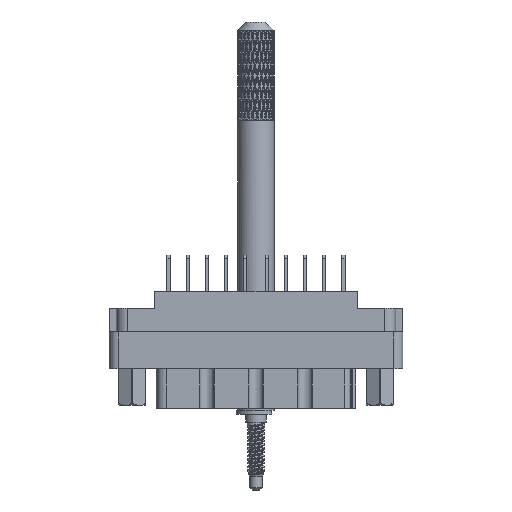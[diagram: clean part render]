
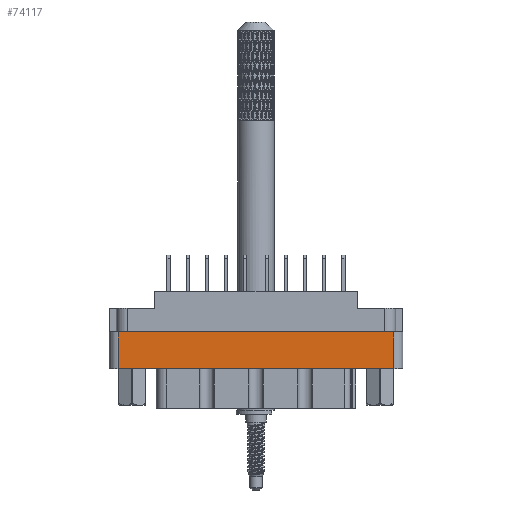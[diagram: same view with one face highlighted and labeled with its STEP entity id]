
A CAD part, front view. The second image highlights one B-rep face of the part: STEP entity #74117.
In plain terms, the highlighted planar face has unit normal (0, -1, 0).
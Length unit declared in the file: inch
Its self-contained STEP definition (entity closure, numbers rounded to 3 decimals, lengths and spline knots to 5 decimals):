
#2895 = VECTOR ( 'NONE', #45526, 39.37008 ) ;
#4321 = DIRECTION ( 'NONE',  ( 0., 0., -1. ) ) ;
#4507 = VERTEX_POINT ( 'NONE', #77688 ) ;
#5155 = CARTESIAN_POINT ( 'NONE',  ( 0.938, -0.438, -0.529 ) ) ;
#8470 = AXIS2_PLACEMENT_3D ( 'NONE', #83076, #100688, #4321 ) ;
#8472 = LINE ( 'NONE', #11501, #2895 ) ;
#9503 = VERTEX_POINT ( 'NONE', #14021 ) ;
#9946 = VERTEX_POINT ( 'NONE', #67772 ) ;
#11501 = CARTESIAN_POINT ( 'NONE',  ( 0., -0.438, -0.529 ) ) ;
#11908 = ORIENTED_EDGE ( 'NONE', *, *, #100642, .F. ) ;
#13003 = DIRECTION ( 'NONE',  ( 1., 0., 0. ) ) ;
#13657 = CARTESIAN_POINT ( 'NONE',  ( 0.938, -0.438, -0.798 ) ) ;
#13785 = CARTESIAN_POINT ( 'NONE',  ( 0., -0.438, -0.277 ) ) ;
#14021 = CARTESIAN_POINT ( 'NONE',  ( 0.938, -0.438, -0.277 ) ) ;
#21577 = PLANE ( 'NONE',  #8470 ) ;
#41378 = FACE_OUTER_BOUND ( 'NONE', #76787, .T. ) ;
#44194 = VECTOR ( 'NONE', #52657, 39.37008 ) ;
#45526 = DIRECTION ( 'NONE',  ( -1., 0., 0. ) ) ;
#49518 = CARTESIAN_POINT ( 'NONE',  ( -0.938, -0.438, -0.798 ) ) ;
#52657 = DIRECTION ( 'NONE',  ( 0., 0., -1. ) ) ;
#55251 = ORIENTED_EDGE ( 'NONE', *, *, #63183, .T. ) ;
#59979 = VECTOR ( 'NONE', #67132, 39.37008 ) ;
#63183 = EDGE_CURVE ( 'NONE', #88322, #9503, #99477, .T. ) ;
#67132 = DIRECTION ( 'NONE',  ( 0., 0., 1. ) ) ;
#67772 = CARTESIAN_POINT ( 'NONE',  ( -0.938, -0.438, -0.277 ) ) ;
#74117 = ADVANCED_FACE ( 'NONE', ( #41378 ), #21577, .T. ) ;
#76787 = EDGE_LOOP ( 'NONE', ( #11908, #105255, #108113, #55251 ) ) ;
#77688 = CARTESIAN_POINT ( 'NONE',  ( -0.938, -0.438, -0.529 ) ) ;
#82447 = LINE ( 'NONE', #49518, #44194 ) ;
#83076 = CARTESIAN_POINT ( 'NONE',  ( -1., -0.438, -0.798 ) ) ;
#83895 = EDGE_CURVE ( 'NONE', #88322, #4507, #8472, .T. ) ;
#86963 = LINE ( 'NONE', #13785, #92444 ) ;
#88322 = VERTEX_POINT ( 'NONE', #5155 ) ;
#92444 = VECTOR ( 'NONE', #13003, 39.37008 ) ;
#99477 = LINE ( 'NONE', #13657, #59979 ) ;
#100642 = EDGE_CURVE ( 'NONE', #9946, #9503, #86963, .T. ) ;
#100688 = DIRECTION ( 'NONE',  ( 0., -1., 0. ) ) ;
#105255 = ORIENTED_EDGE ( 'NONE', *, *, #108707, .T. ) ;
#108113 = ORIENTED_EDGE ( 'NONE', *, *, #83895, .F. ) ;
#108707 = EDGE_CURVE ( 'NONE', #9946, #4507, #82447, .T. ) ;
